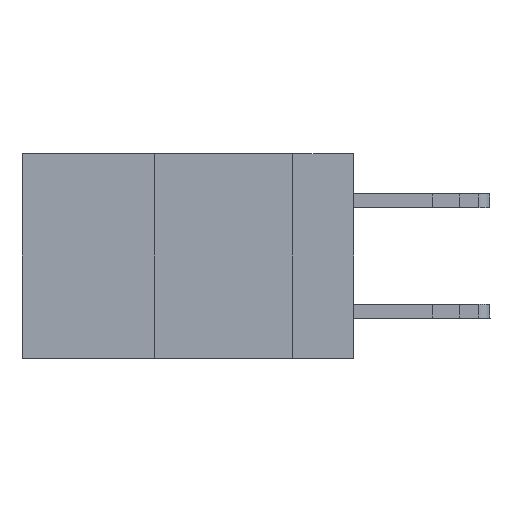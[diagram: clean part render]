
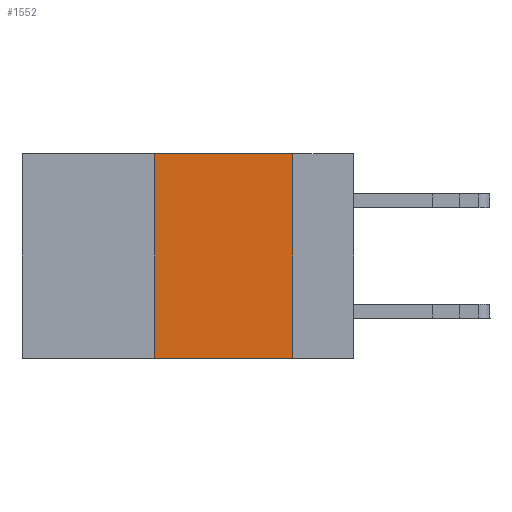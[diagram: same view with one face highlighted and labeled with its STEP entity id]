
A CAD part, left-side view. The second image highlights one B-rep face of the part: STEP entity #1552.
In plain terms, the highlighted planar face has unit normal (-1, 0, 0).
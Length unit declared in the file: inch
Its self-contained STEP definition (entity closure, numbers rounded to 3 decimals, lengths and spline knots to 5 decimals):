
#104 = CARTESIAN_POINT ( 'NONE',  ( 0., 0.6, 0. ) ) ;
#501 = CARTESIAN_POINT ( 'NONE',  ( 0., 0.11, 0. ) ) ;
#1552 = ADVANCED_FACE ( 'NONE', ( #1568 ), #9376, .F. ) ;
#1568 = FACE_OUTER_BOUND ( 'NONE', #15713, .T. ) ;
#1805 = CARTESIAN_POINT ( 'NONE',  ( 0., 0.36, 0. ) ) ;
#2009 = VERTEX_POINT ( 'NONE', #2902 ) ;
#2902 = CARTESIAN_POINT ( 'NONE',  ( 0., 0.36, -0.37 ) ) ;
#3343 = LINE ( 'NONE', #5847, #13526 ) ;
#3377 = CARTESIAN_POINT ( 'NONE',  ( 0., 0.6, -0.37 ) ) ;
#3637 = CARTESIAN_POINT ( 'NONE',  ( 0., 0.11, -0.37 ) ) ;
#4048 = VECTOR ( 'NONE', #14584, 39.37008 ) ;
#4405 = DIRECTION ( 'NONE',  ( 0., -1., 0. ) ) ;
#4424 = DIRECTION ( 'NONE',  ( 0., 0., 1. ) ) ;
#4467 = LINE ( 'NONE', #14084, #11436 ) ;
#5122 = VERTEX_POINT ( 'NONE', #501 ) ;
#5598 = VECTOR ( 'NONE', #7633, 39.37008 ) ;
#5847 = CARTESIAN_POINT ( 'NONE',  ( 0., 0.36, 0. ) ) ;
#6352 = AXIS2_PLACEMENT_3D ( 'NONE', #104, #17055, #16766 ) ;
#6969 = ORIENTED_EDGE ( 'NONE', *, *, #17279, .F. ) ;
#7633 = DIRECTION ( 'NONE',  ( 0., 0., -1. ) ) ;
#9376 = PLANE ( 'NONE',  #6352 ) ;
#11436 = VECTOR ( 'NONE', #4405, 39.37008 ) ;
#11454 = LINE ( 'NONE', #3377, #4048 ) ;
#12134 = EDGE_CURVE ( 'NONE', #5122, #13149, #13374, .T. ) ;
#13149 = VERTEX_POINT ( 'NONE', #3637 ) ;
#13374 = LINE ( 'NONE', #14504, #5598 ) ;
#13526 = VECTOR ( 'NONE', #4424, 39.37008 ) ;
#13861 = ORIENTED_EDGE ( 'NONE', *, *, #12134, .F. ) ;
#14084 = CARTESIAN_POINT ( 'NONE',  ( 0., 0.6, 0. ) ) ;
#14504 = CARTESIAN_POINT ( 'NONE',  ( 0., 0.11, 0. ) ) ;
#14584 = DIRECTION ( 'NONE',  ( 0., -1., 0. ) ) ;
#15441 = EDGE_CURVE ( 'NONE', #2009, #13149, #11454, .T. ) ;
#15713 = EDGE_LOOP ( 'NONE', ( #13861, #17442, #6969, #17853 ) ) ;
#15921 = EDGE_CURVE ( 'NONE', #18016, #5122, #4467, .T. ) ;
#16766 = DIRECTION ( 'NONE',  ( 0., 0., -1. ) ) ;
#17055 = DIRECTION ( 'NONE',  ( 1., 0., 0. ) ) ;
#17279 = EDGE_CURVE ( 'NONE', #2009, #18016, #3343, .T. ) ;
#17442 = ORIENTED_EDGE ( 'NONE', *, *, #15921, .F. ) ;
#17853 = ORIENTED_EDGE ( 'NONE', *, *, #15441, .T. ) ;
#18016 = VERTEX_POINT ( 'NONE', #1805 ) ;
